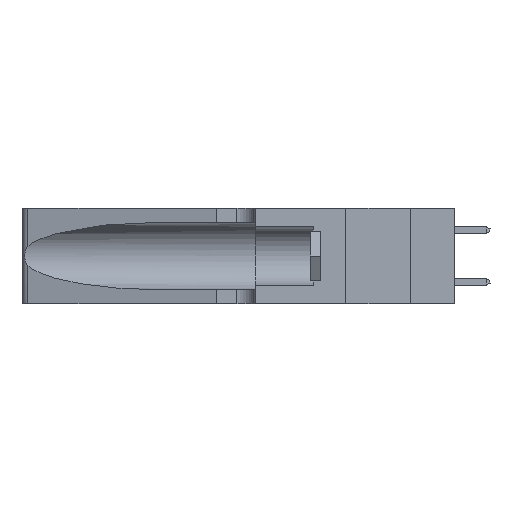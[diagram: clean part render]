
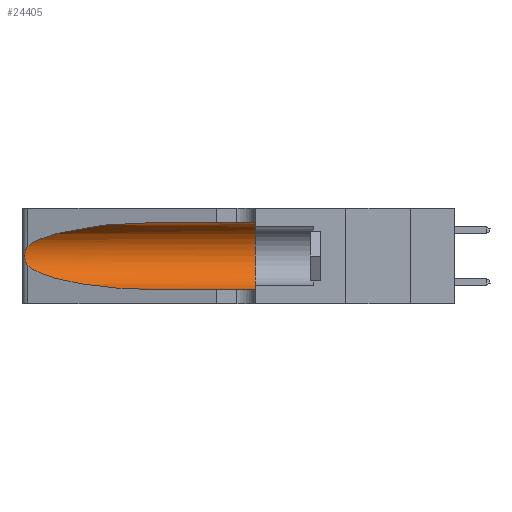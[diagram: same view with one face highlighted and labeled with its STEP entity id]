
A CAD part, left-side view. The second image highlights one B-rep face of the part: STEP entity #24405.
In plain terms, the highlighted cylindrical face has radius 3.308 mm (diameter 6.617 mm), a partial arc.
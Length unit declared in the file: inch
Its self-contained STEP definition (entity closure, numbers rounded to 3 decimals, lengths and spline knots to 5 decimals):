
#608 = DIRECTION ( 'NONE',  ( 0., 1., 0. ) ) ;
#800 = CARTESIAN_POINT ( 'NONE',  ( 0.1305, 0.72297, 0.05475 ) ) ;
#992 = ORIENTED_EDGE ( 'NONE', *, *, #15886, .F. ) ;
#1278 = ORIENTED_EDGE ( 'NONE', *, *, #18367, .F. ) ;
#1416 = CARTESIAN_POINT ( 'NONE',  ( 0.26075, 1.23896, 0.178 ) ) ;
#1442 = CARTESIAN_POINT ( 'NONE',  ( 0.2373, 1.15595, 0.28018 ) ) ;
#1482 = CARTESIAN_POINT ( 'NONE',  ( 0.1305, 1.61858, 0.31525 ) ) ;
#1914 =( BOUNDED_CURVE ( )  B_SPLINE_CURVE ( 3, ( #18849, #3365, #1442, #7068 ),
 .UNSPECIFIED., .F., .F. ) 
 B_SPLINE_CURVE_WITH_KNOTS ( ( 4, 4 ),
 ( 1.5708, 2.84003 ),
 .UNSPECIFIED. ) 
 CURVE ( )  GEOMETRIC_REPRESENTATION_ITEM ( )  RATIONAL_B_SPLINE_CURVE ( ( 1., 0.87, 0.87, 1. ) ) 
 REPRESENTATION_ITEM ( '' )  );
#1969 = CARTESIAN_POINT ( 'NONE',  ( 0.2373, 1.15595, 0.08982 ) ) ;
#2113 = VECTOR ( 'NONE', #19543, 39.37008 ) ;
#3365 = CARTESIAN_POINT ( 'NONE',  ( 0.18966, 0.96281, 0.31525 ) ) ;
#3424 = CARTESIAN_POINT ( 'NONE',  ( 0.25487, 1.22718, 0.14631 ) ) ;
#3977 = CIRCLE ( 'NONE', #7826, 0.13025 ) ;
#4014 = VERTEX_POINT ( 'NONE', #6568 ) ;
#4324 = DIRECTION ( 'NONE',  ( 0., 0., 1. ) ) ;
#4409 = ORIENTED_EDGE ( 'NONE', *, *, #12180, .T. ) ;
#6091 = CARTESIAN_POINT ( 'NONE',  ( 0.25487, 1.22718, 0.14631 ) ) ;
#6388 = VERTEX_POINT ( 'NONE', #9320 ) ;
#6568 = CARTESIAN_POINT ( 'NONE',  ( 0.1305, 0.35, 0.05475 ) ) ;
#6737 = VERTEX_POINT ( 'NONE', #800 ) ;
#7068 = CARTESIAN_POINT ( 'NONE',  ( 0.25487, 1.22718, 0.22369 ) ) ;
#7826 = AXIS2_PLACEMENT_3D ( 'NONE', #10429, #608, #4324 ) ;
#8289 = LINE ( 'NONE', #17558, #2113 ) ;
#8346 = VERTEX_POINT ( 'NONE', #13289 ) ;
#9256 = CARTESIAN_POINT ( 'NONE',  ( 0.26017, 1.23833, 0.17102 ) ) ;
#9319 = VECTOR ( 'NONE', #23264, 39.37008 ) ;
#9320 = CARTESIAN_POINT ( 'NONE',  ( 0.25487, 1.22718, 0.22369 ) ) ;
#10116 = ORIENTED_EDGE ( 'NONE', *, *, #18251, .T. ) ;
#10256 = FACE_OUTER_BOUND ( 'NONE', #19514, .T. ) ;
#10429 = CARTESIAN_POINT ( 'NONE',  ( 0.1305, 0.35, 0.185 ) ) ;
#11060 = CARTESIAN_POINT ( 'NONE',  ( 0.25487, 1.22718, 0.22369 ) ) ;
#11403 = EDGE_CURVE ( 'NONE', #6388, #21127, #23704, .T. ) ;
#12037 = CARTESIAN_POINT ( 'NONE',  ( 0.1305, 0.72297, 0.05475 ) ) ;
#12180 = EDGE_CURVE ( 'NONE', #21127, #6737, #17843, .T. ) ;
#12606 = DIRECTION ( 'NONE',  ( 0., 0., -1. ) ) ;
#12888 = CARTESIAN_POINT ( 'NONE',  ( 0.25787, 1.23484, 0.2124 ) ) ;
#13289 = CARTESIAN_POINT ( 'NONE',  ( 0.1305, 0.72297, 0.31525 ) ) ;
#13408 = CARTESIAN_POINT ( 'NONE',  ( 0.25487, 1.22718, 0.14631 ) ) ;
#13903 = EDGE_CURVE ( 'NONE', #8346, #6388, #1914, .T. ) ;
#14903 = CARTESIAN_POINT ( 'NONE',  ( 0.25639, 1.23186, 0.15144 ) ) ;
#14991 = CARTESIAN_POINT ( 'NONE',  ( 0.25639, 1.23184, 0.21858 ) ) ;
#15237 = CARTESIAN_POINT ( 'NONE',  ( 0.25555, 1.22993, 0.14849 ) ) ;
#15241 = AXIS2_PLACEMENT_3D ( 'NONE', #18477, #18563, #12606 ) ;
#15781 = CARTESIAN_POINT ( 'NONE',  ( 0.18966, 0.96281, 0.05475 ) ) ;
#15886 = EDGE_CURVE ( 'NONE', #8346, #25002, #19781, .T. ) ;
#16510 = ORIENTED_EDGE ( 'NONE', *, *, #13903, .T. ) ;
#16938 = CARTESIAN_POINT ( 'NONE',  ( 0.25854, 1.2359, 0.20912 ) ) ;
#17083 = CARTESIAN_POINT ( 'NONE',  ( 0.25555, 1.22994, 0.2215 ) ) ;
#17169 = CARTESIAN_POINT ( 'NONE',  ( 0.26018, 1.23835, 0.19895 ) ) ;
#17558 = CARTESIAN_POINT ( 'NONE',  ( 0.1305, 1.61858, 0.05475 ) ) ;
#17843 =( BOUNDED_CURVE ( )  B_SPLINE_CURVE ( 3, ( #6091, #1969, #15781, #12037 ),
 .UNSPECIFIED., .F., .F. ) 
 B_SPLINE_CURVE_WITH_KNOTS ( ( 4, 4 ),
 ( 3.44316, 4.71239 ),
 .UNSPECIFIED. ) 
 CURVE ( )  GEOMETRIC_REPRESENTATION_ITEM ( )  RATIONAL_B_SPLINE_CURVE ( ( 1., 0.87, 0.87, 1. ) ) 
 REPRESENTATION_ITEM ( '' )  );
#18251 = EDGE_CURVE ( 'NONE', #6737, #4014, #8289, .T. ) ;
#18367 = EDGE_CURVE ( 'NONE', #25002, #4014, #3977, .T. ) ;
#18477 = CARTESIAN_POINT ( 'NONE',  ( 0.1305, 1.61858, 0.185 ) ) ;
#18563 = DIRECTION ( 'NONE',  ( 0., -1., 0. ) ) ;
#18849 = CARTESIAN_POINT ( 'NONE',  ( 0.1305, 0.72297, 0.31525 ) ) ;
#18909 = CARTESIAN_POINT ( 'NONE',  ( 0.26075, 1.23896, 0.19203 ) ) ;
#19085 = CARTESIAN_POINT ( 'NONE',  ( 0.25856, 1.23593, 0.16098 ) ) ;
#19514 = EDGE_LOOP ( 'NONE', ( #16510, #20016, #4409, #10116, #1278, #992 ) ) ;
#19543 = DIRECTION ( 'NONE',  ( 0., -1., 0. ) ) ;
#19781 = LINE ( 'NONE', #1482, #9319 ) ;
#20016 = ORIENTED_EDGE ( 'NONE', *, *, #11403, .T. ) ;
#20743 = CYLINDRICAL_SURFACE ( 'NONE', #15241, 0.13025 ) ;
#21065 = CARTESIAN_POINT ( 'NONE',  ( 0.25789, 1.23486, 0.15765 ) ) ;
#21127 = VERTEX_POINT ( 'NONE', #13408 ) ;
#21977 = CARTESIAN_POINT ( 'NONE',  ( 0.1305, 0.35, 0.31525 ) ) ;
#23264 = DIRECTION ( 'NONE',  ( 0., -1., 0. ) ) ;
#23704 = B_SPLINE_CURVE_WITH_KNOTS ( 'NONE', 3,
 ( #11060, #17083, #14991, #12888, #16938, #17169, #18909, #1416, #9256, #19085, #21065, #14903, #15237, #3424 ),
 .UNSPECIFIED., .F., .F.,
 ( 4, 2, 2, 2, 2, 2, 4 ),
 ( 0., 0.00027, 0.00053, 0.00107, 0.0016, 0.00187, 0.00214 ),
 .UNSPECIFIED. ) ;
#24405 = ADVANCED_FACE ( 'NONE', ( #10256 ), #20743, .F. ) ;
#25002 = VERTEX_POINT ( 'NONE', #21977 ) ;
